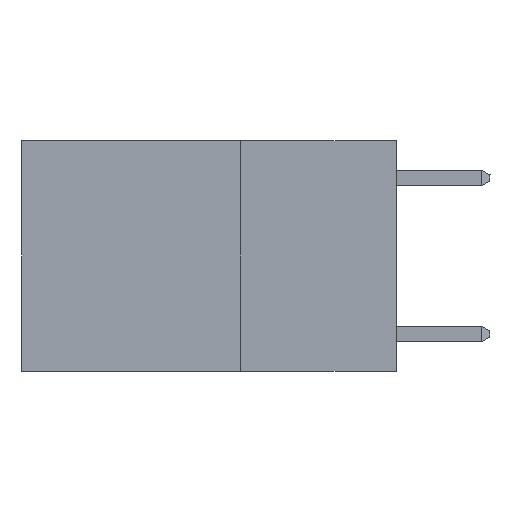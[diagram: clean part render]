
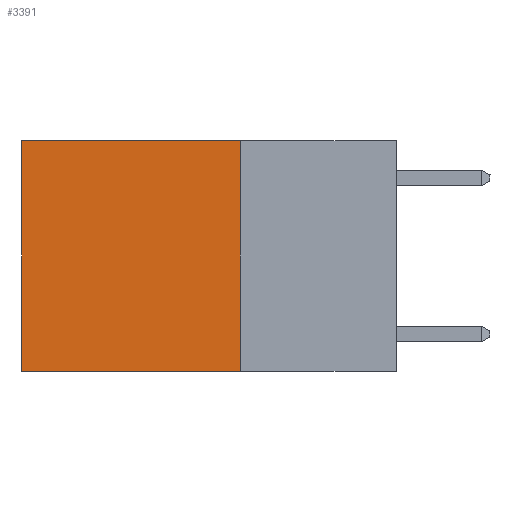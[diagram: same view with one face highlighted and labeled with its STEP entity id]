
A CAD part, left-side view. The second image highlights one B-rep face of the part: STEP entity #3391.
In plain terms, the highlighted planar face has unit normal (-1, 0, 0).
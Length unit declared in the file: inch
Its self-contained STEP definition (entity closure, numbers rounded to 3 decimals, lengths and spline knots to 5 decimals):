
#87 = DIRECTION ( 'NONE',  ( 0., 0., -1. ) ) ;
#447 = LINE ( 'NONE', #2424, #6182 ) ;
#709 = CARTESIAN_POINT ( 'NONE',  ( 0.2625, 0.6, 0. ) ) ;
#782 = LINE ( 'NONE', #6708, #6167 ) ;
#1346 = FACE_OUTER_BOUND ( 'NONE', #3362, .T. ) ;
#1634 = DIRECTION ( 'NONE',  ( 1., 0., 0. ) ) ;
#2403 = CARTESIAN_POINT ( 'NONE',  ( 0.2625, 0.6, 0. ) ) ;
#2424 = CARTESIAN_POINT ( 'NONE',  ( 0.2625, 0.25, 0. ) ) ;
#2484 = VERTEX_POINT ( 'NONE', #2403 ) ;
#3362 = EDGE_LOOP ( 'NONE', ( #6038, #3608, #3880, #10964 ) ) ;
#3384 = LINE ( 'NONE', #12658, #9139 ) ;
#3391 = ADVANCED_FACE ( 'NONE', ( #1346 ), #14032, .F. ) ;
#3608 = ORIENTED_EDGE ( 'NONE', *, *, #6228, .F. ) ;
#3880 = ORIENTED_EDGE ( 'NONE', *, *, #12950, .F. ) ;
#4179 = EDGE_CURVE ( 'NONE', #9775, #2484, #782, .T. ) ;
#5556 = CARTESIAN_POINT ( 'NONE',  ( 0.2625, 0.6, -0.37 ) ) ;
#6038 = ORIENTED_EDGE ( 'NONE', *, *, #12467, .T. ) ;
#6167 = VECTOR ( 'NONE', #7853, 39.37008 ) ;
#6182 = VECTOR ( 'NONE', #87, 39.37008 ) ;
#6228 = EDGE_CURVE ( 'NONE', #7395, #10681, #3384, .T. ) ;
#6328 = LINE ( 'NONE', #709, #12326 ) ;
#6708 = CARTESIAN_POINT ( 'NONE',  ( 0.2625, 0.25, 0. ) ) ;
#7346 = CARTESIAN_POINT ( 'NONE',  ( 0.2625, 0.25, 0. ) ) ;
#7395 = VERTEX_POINT ( 'NONE', #11012 ) ;
#7853 = DIRECTION ( 'NONE',  ( 0., 1., 0. ) ) ;
#9139 = VECTOR ( 'NONE', #13759, 39.37008 ) ;
#9630 = DIRECTION ( 'NONE',  ( 0., 0., -1. ) ) ;
#9775 = VERTEX_POINT ( 'NONE', #10838 ) ;
#9856 = DIRECTION ( 'NONE',  ( 0., 0., -1. ) ) ;
#10681 = VERTEX_POINT ( 'NONE', #5556 ) ;
#10838 = CARTESIAN_POINT ( 'NONE',  ( 0.2625, 0.25, 0. ) ) ;
#10964 = ORIENTED_EDGE ( 'NONE', *, *, #4179, .T. ) ;
#11012 = CARTESIAN_POINT ( 'NONE',  ( 0.2625, 0.25, -0.37 ) ) ;
#11728 = AXIS2_PLACEMENT_3D ( 'NONE', #7346, #1634, #9630 ) ;
#12326 = VECTOR ( 'NONE', #9856, 39.37008 ) ;
#12467 = EDGE_CURVE ( 'NONE', #2484, #10681, #6328, .T. ) ;
#12658 = CARTESIAN_POINT ( 'NONE',  ( 0.2625, 0.25, -0.37 ) ) ;
#12950 = EDGE_CURVE ( 'NONE', #9775, #7395, #447, .T. ) ;
#13759 = DIRECTION ( 'NONE',  ( 0., 1., 0. ) ) ;
#14032 = PLANE ( 'NONE',  #11728 ) ;
